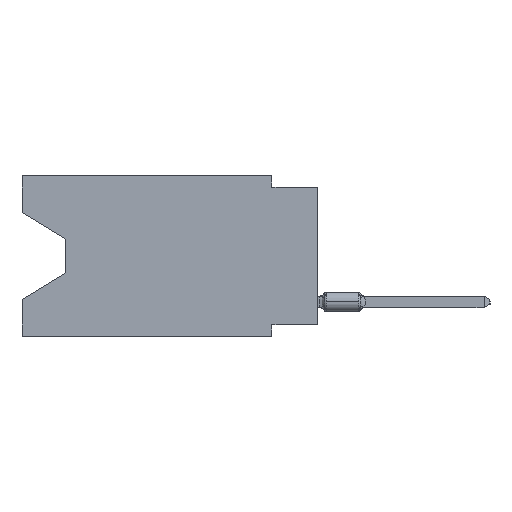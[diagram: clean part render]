
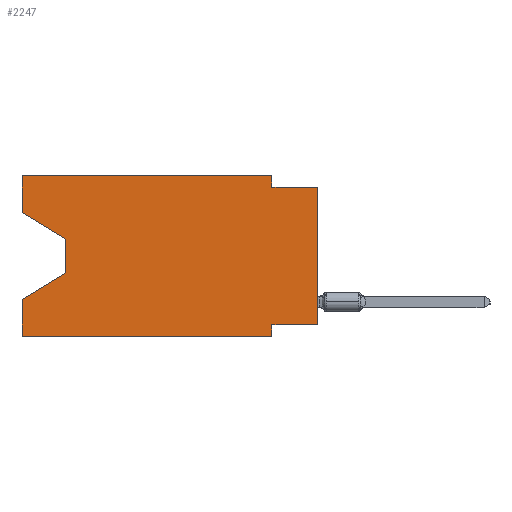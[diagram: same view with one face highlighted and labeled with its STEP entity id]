
A CAD part, left-side view. The second image highlights one B-rep face of the part: STEP entity #2247.
In plain terms, the highlighted planar face has unit normal (-1, 0, 0).
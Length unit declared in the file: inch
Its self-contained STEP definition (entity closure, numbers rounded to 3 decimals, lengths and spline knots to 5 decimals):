
#1623 = CARTESIAN_POINT ( 'NONE',  ( 0., 0.645, -0.08025 ) ) ;
#2247 = ADVANCED_FACE ( 'NONE', ( #9364 ), #29889, .F. ) ;
#2976 = DIRECTION ( 'NONE',  ( 0., -0.855, -0.519 ) ) ;
#3706 = CARTESIAN_POINT ( 'NONE',  ( 0., 0., -0.325 ) ) ;
#3978 = EDGE_CURVE ( 'NONE', #20959, #39328, #28389, .T. ) ;
#4873 = CARTESIAN_POINT ( 'NONE',  ( 0., 0.645, -0.08025 ) ) ;
#5054 = VERTEX_POINT ( 'NONE', #15512 ) ;
#5604 = LINE ( 'NONE', #30568, #31009 ) ;
#5843 = EDGE_CURVE ( 'NONE', #20959, #14541, #6952, .T. ) ;
#5943 = LINE ( 'NONE', #27094, #20770 ) ;
#6952 = LINE ( 'NONE', #29078, #29584 ) ;
#6989 = VERTEX_POINT ( 'NONE', #8644 ) ;
#7747 = CARTESIAN_POINT ( 'NONE',  ( 0., 0.55, -0.138 ) ) ;
#8040 = AXIS2_PLACEMENT_3D ( 'NONE', #21424, #33489, #24627 ) ;
#8087 = DIRECTION ( 'NONE',  ( 0., 0., 1. ) ) ;
#8393 = CARTESIAN_POINT ( 'NONE',  ( 0., 0.1, 0. ) ) ;
#8460 = ORIENTED_EDGE ( 'NONE', *, *, #10718, .F. ) ;
#8644 = CARTESIAN_POINT ( 'NONE',  ( 0., 0., -0.325 ) ) ;
#8846 = DIRECTION ( 'NONE',  ( 0., -1., 0. ) ) ;
#8862 = ORIENTED_EDGE ( 'NONE', *, *, #14811, .F. ) ;
#9364 = FACE_OUTER_BOUND ( 'NONE', #11919, .T. ) ;
#9800 = DIRECTION ( 'NONE',  ( 0., 0., 1. ) ) ;
#10017 = CARTESIAN_POINT ( 'NONE',  ( 0., 0.645, 0. ) ) ;
#10718 = EDGE_CURVE ( 'NONE', #14541, #27586, #5604, .T. ) ;
#10914 = CARTESIAN_POINT ( 'NONE',  ( 0., 0.1, -0.025 ) ) ;
#11016 = VERTEX_POINT ( 'NONE', #14214 ) ;
#11091 = VECTOR ( 'NONE', #8087, 39.37008 ) ;
#11919 = EDGE_LOOP ( 'NONE', ( #23794, #18721, #34906, #8862, #26222, #23032, #16161, #16561, #23070, #29931, #8460, #12105 ) ) ;
#12105 = ORIENTED_EDGE ( 'NONE', *, *, #5843, .F. ) ;
#13603 = EDGE_CURVE ( 'NONE', #6989, #22779, #36255, .T. ) ;
#13683 = VECTOR ( 'NONE', #37724, 39.37008 ) ;
#13709 = LINE ( 'NONE', #25993, #20174 ) ;
#14214 = CARTESIAN_POINT ( 'NONE',  ( 0., 0.1, -0.325 ) ) ;
#14467 = VERTEX_POINT ( 'NONE', #25723 ) ;
#14541 = VERTEX_POINT ( 'NONE', #34994 ) ;
#14811 = EDGE_CURVE ( 'NONE', #5054, #23646, #18664, .T. ) ;
#15317 = EDGE_CURVE ( 'NONE', #14467, #23646, #19801, .T. ) ;
#15351 = CARTESIAN_POINT ( 'NONE',  ( 0., 0.645, -0.26975 ) ) ;
#15512 = CARTESIAN_POINT ( 'NONE',  ( 0., 0.645, -0.35 ) ) ;
#15607 = DIRECTION ( 'NONE',  ( 0., -1., 0. ) ) ;
#16161 = ORIENTED_EDGE ( 'NONE', *, *, #35990, .F. ) ;
#16414 = EDGE_CURVE ( 'NONE', #39328, #14467, #35327, .T. ) ;
#16561 = ORIENTED_EDGE ( 'NONE', *, *, #13603, .T. ) ;
#17018 = DIRECTION ( 'NONE',  ( 0., 0., -1. ) ) ;
#17185 = CARTESIAN_POINT ( 'NONE',  ( 0., 0.55, -0.212 ) ) ;
#18288 = VECTOR ( 'NONE', #20215, 39.37008 ) ;
#18324 = CARTESIAN_POINT ( 'NONE',  ( 0., 0., -0.025 ) ) ;
#18664 = LINE ( 'NONE', #10017, #24055 ) ;
#18721 = ORIENTED_EDGE ( 'NONE', *, *, #16414, .T. ) ;
#19801 = LINE ( 'NONE', #17185, #18288 ) ;
#20174 = VECTOR ( 'NONE', #38262, 39.37008 ) ;
#20215 = DIRECTION ( 'NONE',  ( 0., 0.855, -0.519 ) ) ;
#20770 = VECTOR ( 'NONE', #15607, 39.37008 ) ;
#20959 = VERTEX_POINT ( 'NONE', #4873 ) ;
#21424 = CARTESIAN_POINT ( 'NONE',  ( 0., 0.645, 0. ) ) ;
#22030 = CARTESIAN_POINT ( 'NONE',  ( 0., 0.1, -0.35 ) ) ;
#22374 = VERTEX_POINT ( 'NONE', #37462 ) ;
#22779 = VERTEX_POINT ( 'NONE', #18324 ) ;
#23032 = ORIENTED_EDGE ( 'NONE', *, *, #39241, .F. ) ;
#23070 = ORIENTED_EDGE ( 'NONE', *, *, #39129, .F. ) ;
#23100 = EDGE_CURVE ( 'NONE', #27586, #33056, #30509, .T. ) ;
#23646 = VERTEX_POINT ( 'NONE', #15351 ) ;
#23794 = ORIENTED_EDGE ( 'NONE', *, *, #3978, .T. ) ;
#24055 = VECTOR ( 'NONE', #9800, 39.37008 ) ;
#24627 = DIRECTION ( 'NONE',  ( 0., 0., -1. ) ) ;
#25041 = DIRECTION ( 'NONE',  ( 0., 1., 0. ) ) ;
#25723 = CARTESIAN_POINT ( 'NONE',  ( 0., 0.55, -0.212 ) ) ;
#25993 = CARTESIAN_POINT ( 'NONE',  ( 0., 0.645, -0.35 ) ) ;
#26222 = ORIENTED_EDGE ( 'NONE', *, *, #37770, .T. ) ;
#26693 = VECTOR ( 'NONE', #17018, 39.37008 ) ;
#27094 = CARTESIAN_POINT ( 'NONE',  ( 0., 0., -0.025 ) ) ;
#27586 = VERTEX_POINT ( 'NONE', #8393 ) ;
#28088 = LINE ( 'NONE', #3706, #29103 ) ;
#28389 = LINE ( 'NONE', #1623, #38446 ) ;
#28477 = CARTESIAN_POINT ( 'NONE',  ( 0., 0.55, -0.138 ) ) ;
#28868 = LINE ( 'NONE', #22030, #13683 ) ;
#29078 = CARTESIAN_POINT ( 'NONE',  ( 0., 0.645, 0. ) ) ;
#29103 = VECTOR ( 'NONE', #25041, 39.37008 ) ;
#29584 = VECTOR ( 'NONE', #35312, 39.37008 ) ;
#29889 = PLANE ( 'NONE',  #8040 ) ;
#29931 = ORIENTED_EDGE ( 'NONE', *, *, #23100, .F. ) ;
#30509 = LINE ( 'NONE', #30708, #31122 ) ;
#30568 = CARTESIAN_POINT ( 'NONE',  ( 0., 0.645, 0. ) ) ;
#30708 = CARTESIAN_POINT ( 'NONE',  ( 0., 0.1, 0. ) ) ;
#31009 = VECTOR ( 'NONE', #8846, 39.37008 ) ;
#31122 = VECTOR ( 'NONE', #33727, 39.37008 ) ;
#33056 = VERTEX_POINT ( 'NONE', #10914 ) ;
#33489 = DIRECTION ( 'NONE',  ( 1., 0., 0. ) ) ;
#33727 = DIRECTION ( 'NONE',  ( 0., 0., -1. ) ) ;
#34906 = ORIENTED_EDGE ( 'NONE', *, *, #15317, .T. ) ;
#34994 = CARTESIAN_POINT ( 'NONE',  ( 0., 0.645, 0. ) ) ;
#35312 = DIRECTION ( 'NONE',  ( 0., 0., 1. ) ) ;
#35327 = LINE ( 'NONE', #7747, #26693 ) ;
#35990 = EDGE_CURVE ( 'NONE', #6989, #11016, #28088, .T. ) ;
#36047 = CARTESIAN_POINT ( 'NONE',  ( 0., 0., 0. ) ) ;
#36255 = LINE ( 'NONE', #36047, #11091 ) ;
#37462 = CARTESIAN_POINT ( 'NONE',  ( 0., 0.1, -0.35 ) ) ;
#37724 = DIRECTION ( 'NONE',  ( 0., 0., -1. ) ) ;
#37770 = EDGE_CURVE ( 'NONE', #5054, #22374, #13709, .T. ) ;
#38262 = DIRECTION ( 'NONE',  ( 0., -1., 0. ) ) ;
#38446 = VECTOR ( 'NONE', #2976, 39.37008 ) ;
#39129 = EDGE_CURVE ( 'NONE', #33056, #22779, #5943, .T. ) ;
#39241 = EDGE_CURVE ( 'NONE', #11016, #22374, #28868, .T. ) ;
#39328 = VERTEX_POINT ( 'NONE', #28477 ) ;
